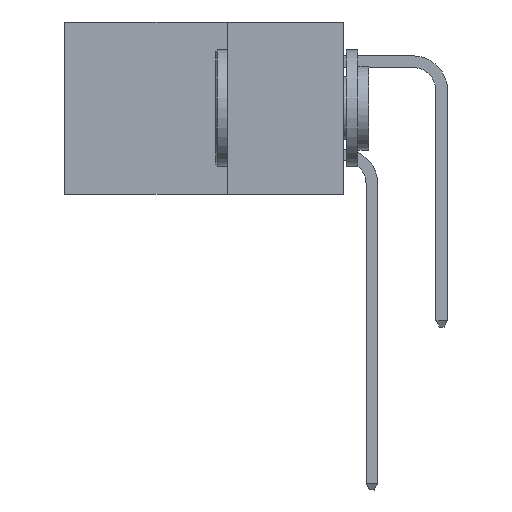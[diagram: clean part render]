
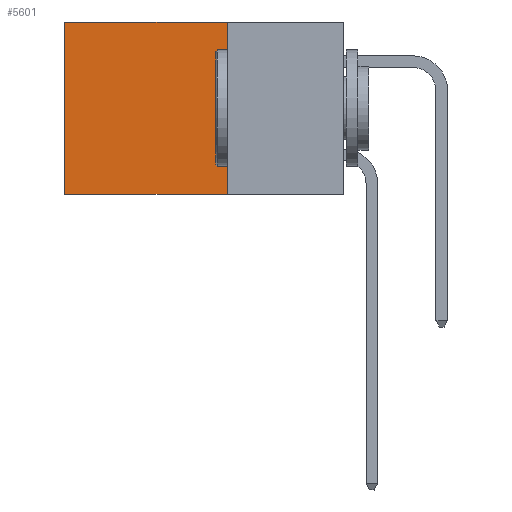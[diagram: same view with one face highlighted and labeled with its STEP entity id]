
A CAD part, left-side view. The second image highlights one B-rep face of the part: STEP entity #5601.
In plain terms, the highlighted planar face has unit normal (-1, 0, 0).
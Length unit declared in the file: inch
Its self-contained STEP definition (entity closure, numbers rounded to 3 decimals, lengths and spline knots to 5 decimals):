
#260 = DIRECTION ( 'NONE',  ( 0., 0., -1. ) ) ;
#424 = LINE ( 'NONE', #5329, #8906 ) ;
#741 = EDGE_CURVE ( 'NONE', #11673, #1873, #10173, .T. ) ;
#789 = VECTOR ( 'NONE', #3489, 39.37008 ) ;
#1381 = CARTESIAN_POINT ( 'NONE',  ( 0.2615, 0.6, -0.37 ) ) ;
#1617 = DIRECTION ( 'NONE',  ( 1., 0., 0. ) ) ;
#1670 = CARTESIAN_POINT ( 'NONE',  ( 0.2615, 0.25, -0.37 ) ) ;
#1873 = VERTEX_POINT ( 'NONE', #1670 ) ;
#2894 = DIRECTION ( 'NONE',  ( 0., 1., 0. ) ) ;
#3008 = EDGE_CURVE ( 'NONE', #7105, #3661, #4064, .T. ) ;
#3489 = DIRECTION ( 'NONE',  ( 0., 1., 0. ) ) ;
#3587 = AXIS2_PLACEMENT_3D ( 'NONE', #14881, #1617, #6598 ) ;
#3661 = VERTEX_POINT ( 'NONE', #3944 ) ;
#3944 = CARTESIAN_POINT ( 'NONE',  ( 0.2615, 0.6, -0.37 ) ) ;
#4064 = LINE ( 'NONE', #1381, #5324 ) ;
#4096 = EDGE_LOOP ( 'NONE', ( #11044, #8101, #6948, #9058 ) ) ;
#4720 = LINE ( 'NONE', #6098, #789 ) ;
#4798 = PLANE ( 'NONE',  #3587 ) ;
#5324 = VECTOR ( 'NONE', #6273, 39.37008 ) ;
#5329 = CARTESIAN_POINT ( 'NONE',  ( 0.2615, 0.25, -0.37 ) ) ;
#5601 = ADVANCED_FACE ( 'NONE', ( #7418 ), #4798, .F. ) ;
#6098 = CARTESIAN_POINT ( 'NONE',  ( 0.2615, 0.25, 0. ) ) ;
#6273 = DIRECTION ( 'NONE',  ( 0., 0., -1. ) ) ;
#6451 = VECTOR ( 'NONE', #260, 39.37008 ) ;
#6598 = DIRECTION ( 'NONE',  ( 0., 0., -1. ) ) ;
#6948 = ORIENTED_EDGE ( 'NONE', *, *, #741, .F. ) ;
#7105 = VERTEX_POINT ( 'NONE', #12173 ) ;
#7418 = FACE_OUTER_BOUND ( 'NONE', #4096, .T. ) ;
#8101 = ORIENTED_EDGE ( 'NONE', *, *, #15523, .F. ) ;
#8759 = CARTESIAN_POINT ( 'NONE',  ( 0.2615, 0.25, 0. ) ) ;
#8906 = VECTOR ( 'NONE', #2894, 39.37008 ) ;
#9058 = ORIENTED_EDGE ( 'NONE', *, *, #13662, .T. ) ;
#10173 = LINE ( 'NONE', #15107, #6451 ) ;
#11044 = ORIENTED_EDGE ( 'NONE', *, *, #3008, .T. ) ;
#11673 = VERTEX_POINT ( 'NONE', #8759 ) ;
#12173 = CARTESIAN_POINT ( 'NONE',  ( 0.2615, 0.6, 0. ) ) ;
#13662 = EDGE_CURVE ( 'NONE', #11673, #7105, #4720, .T. ) ;
#14881 = CARTESIAN_POINT ( 'NONE',  ( 0.2615, 0.25, -0.37 ) ) ;
#15107 = CARTESIAN_POINT ( 'NONE',  ( 0.2615, 0.25, -0.37 ) ) ;
#15523 = EDGE_CURVE ( 'NONE', #1873, #3661, #424, .T. ) ;
